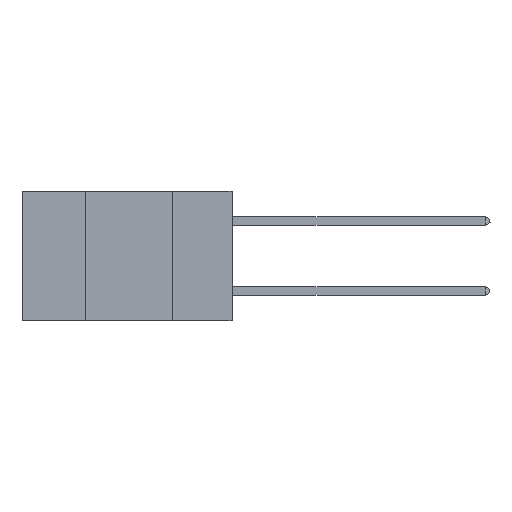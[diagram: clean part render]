
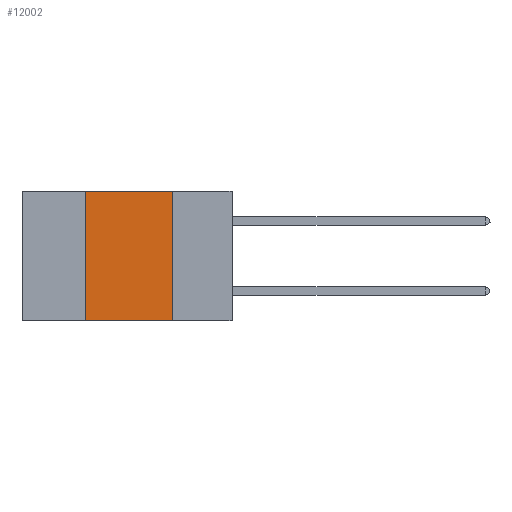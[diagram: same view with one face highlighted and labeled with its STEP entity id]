
A CAD part, left-side view. The second image highlights one B-rep face of the part: STEP entity #12002.
In plain terms, the highlighted planar face has unit normal (-1, 0, 0).
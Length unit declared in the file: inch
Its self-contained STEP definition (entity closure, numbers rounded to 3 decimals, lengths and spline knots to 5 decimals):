
#242 = PLANE ( 'NONE',  #6306 ) ;
#250 = CARTESIAN_POINT ( 'NONE',  ( 0., 0.17, 0. ) ) ;
#496 = VERTEX_POINT ( 'NONE', #602 ) ;
#602 = CARTESIAN_POINT ( 'NONE',  ( 0., 0.42, 0. ) ) ;
#665 = CARTESIAN_POINT ( 'NONE',  ( 0., 0.42, -0.37 ) ) ;
#1097 = LINE ( 'NONE', #10449, #3195 ) ;
#1214 = DIRECTION ( 'NONE',  ( 1., 0., 0. ) ) ;
#1239 = EDGE_CURVE ( 'NONE', #1842, #2524, #6684, .T. ) ;
#1302 = ORIENTED_EDGE ( 'NONE', *, *, #1239, .T. ) ;
#1544 = EDGE_CURVE ( 'NONE', #1842, #496, #6651, .T. ) ;
#1842 = VERTEX_POINT ( 'NONE', #665 ) ;
#2083 = DIRECTION ( 'NONE',  ( 0., 0., -1. ) ) ;
#2114 = CARTESIAN_POINT ( 'NONE',  ( 0., 0.6, -0.37 ) ) ;
#2152 = EDGE_CURVE ( 'NONE', #496, #3300, #6204, .T. ) ;
#2524 = VERTEX_POINT ( 'NONE', #7786 ) ;
#2556 = ORIENTED_EDGE ( 'NONE', *, *, #2152, .F. ) ;
#3054 = CARTESIAN_POINT ( 'NONE',  ( 0., 0.6, 0. ) ) ;
#3195 = VECTOR ( 'NONE', #2083, 39.37008 ) ;
#3300 = VERTEX_POINT ( 'NONE', #250 ) ;
#4069 = VECTOR ( 'NONE', #10420, 39.37008 ) ;
#4096 = CARTESIAN_POINT ( 'NONE',  ( 0., 0.6, 0. ) ) ;
#4709 = FACE_OUTER_BOUND ( 'NONE', #9382, .T. ) ;
#4946 = DIRECTION ( 'NONE',  ( 0., 0., -1. ) ) ;
#5001 = DIRECTION ( 'NONE',  ( 0., -1., 0. ) ) ;
#5039 = VECTOR ( 'NONE', #11076, 39.37008 ) ;
#6204 = LINE ( 'NONE', #4096, #6760 ) ;
#6306 = AXIS2_PLACEMENT_3D ( 'NONE', #3054, #1214, #4946 ) ;
#6651 = LINE ( 'NONE', #11366, #5039 ) ;
#6684 = LINE ( 'NONE', #2114, #4069 ) ;
#6760 = VECTOR ( 'NONE', #5001, 39.37008 ) ;
#7786 = CARTESIAN_POINT ( 'NONE',  ( 0., 0.17, -0.37 ) ) ;
#9113 = ORIENTED_EDGE ( 'NONE', *, *, #1544, .F. ) ;
#9382 = EDGE_LOOP ( 'NONE', ( #11517, #2556, #9113, #1302 ) ) ;
#10420 = DIRECTION ( 'NONE',  ( 0., -1., 0. ) ) ;
#10449 = CARTESIAN_POINT ( 'NONE',  ( 0., 0.17, 0. ) ) ;
#11076 = DIRECTION ( 'NONE',  ( 0., 0., 1. ) ) ;
#11366 = CARTESIAN_POINT ( 'NONE',  ( 0., 0.42, 0. ) ) ;
#11517 = ORIENTED_EDGE ( 'NONE', *, *, #11939, .F. ) ;
#11939 = EDGE_CURVE ( 'NONE', #3300, #2524, #1097, .T. ) ;
#12002 = ADVANCED_FACE ( 'NONE', ( #4709 ), #242, .F. ) ;
